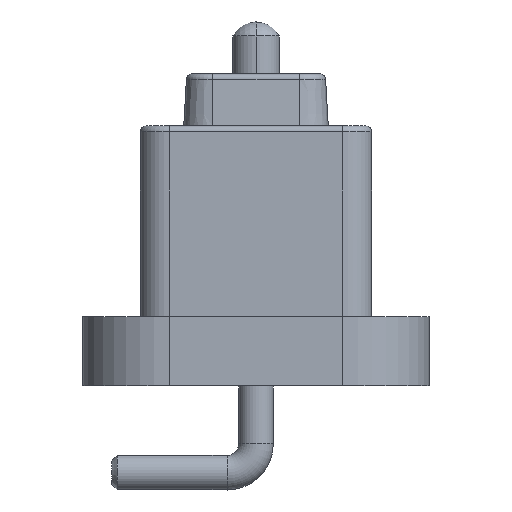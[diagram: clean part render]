
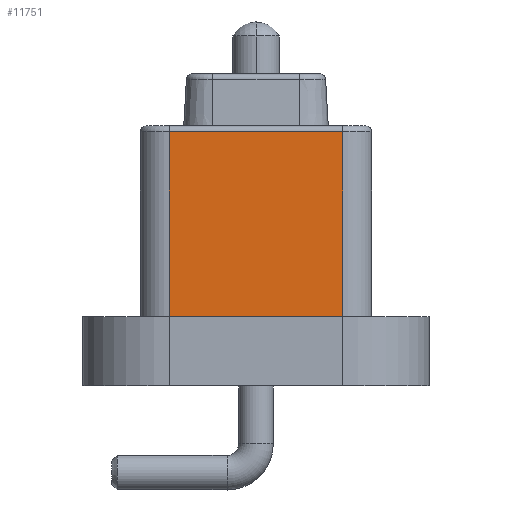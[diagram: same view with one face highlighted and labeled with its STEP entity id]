
A CAD part, left-side view. The second image highlights one B-rep face of the part: STEP entity #11751.
In plain terms, the highlighted planar face has unit normal (-1, 0, 0).
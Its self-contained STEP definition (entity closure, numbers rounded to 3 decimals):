
#188 = CARTESIAN_POINT ( 'NONE',  ( -8.45, -1.5, -0.1 ) ) ;
#852 = PLANE ( 'NONE',  #7900 ) ;
#1420 = VERTEX_POINT ( 'NONE', #5908 ) ;
#2138 = LINE ( 'NONE', #5866, #3477 ) ;
#2346 = LINE ( 'NONE', #188, #6179 ) ;
#3477 = VECTOR ( 'NONE', #9579, 1000. ) ;
#3479 = ORIENTED_EDGE ( 'NONE', *, *, #7312, .T. ) ;
#3485 = CARTESIAN_POINT ( 'NONE',  ( -8.45, 1.5, -0.1 ) ) ;
#3755 = LINE ( 'NONE', #6611, #8312 ) ;
#4085 = ORIENTED_EDGE ( 'NONE', *, *, #5429, .T. ) ;
#4797 = DIRECTION ( 'NONE',  ( 0., 1., 0. ) ) ;
#5429 = EDGE_CURVE ( 'NONE', #1420, #5459, #3755, .T. ) ;
#5459 = VERTEX_POINT ( 'NONE', #8450 ) ;
#5800 = CARTESIAN_POINT ( 'NONE',  ( -8.45, 1.5, -0.1 ) ) ;
#5804 = CARTESIAN_POINT ( 'NONE',  ( -8.45, 0., -1.7 ) ) ;
#5808 = DIRECTION ( 'NONE',  ( 0., 0., 1. ) ) ;
#5866 = CARTESIAN_POINT ( 'NONE',  ( -8.45, 1.5, -3.3 ) ) ;
#5908 = CARTESIAN_POINT ( 'NONE',  ( -8.45, -1.5, -3.3 ) ) ;
#6064 = DIRECTION ( 'NONE',  ( 0., 1., 0. ) ) ;
#6179 = VECTOR ( 'NONE', #6064, 1000. ) ;
#6319 = CARTESIAN_POINT ( 'NONE',  ( -8.45, 1.5, -3.3 ) ) ;
#6611 = CARTESIAN_POINT ( 'NONE',  ( -8.45, -1.5, -3.3 ) ) ;
#7011 = EDGE_CURVE ( 'NONE', #5459, #8961, #2346, .T. ) ;
#7312 = EDGE_CURVE ( 'NONE', #11489, #1420, #2138, .T. ) ;
#7433 = VECTOR ( 'NONE', #11280, 1000. ) ;
#7900 = AXIS2_PLACEMENT_3D ( 'NONE', #5804, #11468, #4797 ) ;
#7980 = EDGE_CURVE ( 'NONE', #8961, #11489, #9344, .T. ) ;
#8312 = VECTOR ( 'NONE', #5808, 1000. ) ;
#8450 = CARTESIAN_POINT ( 'NONE',  ( -8.45, -1.5, -0.1 ) ) ;
#8961 = VERTEX_POINT ( 'NONE', #5800 ) ;
#9067 = EDGE_LOOP ( 'NONE', ( #11068, #3479, #4085, #11905 ) ) ;
#9344 = LINE ( 'NONE', #3485, #7433 ) ;
#9579 = DIRECTION ( 'NONE',  ( 0., -1., 0. ) ) ;
#11061 = FACE_OUTER_BOUND ( 'NONE', #9067, .T. ) ;
#11068 = ORIENTED_EDGE ( 'NONE', *, *, #7980, .T. ) ;
#11280 = DIRECTION ( 'NONE',  ( 0., 0., -1. ) ) ;
#11468 = DIRECTION ( 'NONE',  ( 1., 0., 0. ) ) ;
#11489 = VERTEX_POINT ( 'NONE', #6319 ) ;
#11751 = ADVANCED_FACE ( 'NONE', ( #11061 ), #852, .F. ) ;
#11905 = ORIENTED_EDGE ( 'NONE', *, *, #7011, .T. ) ;
